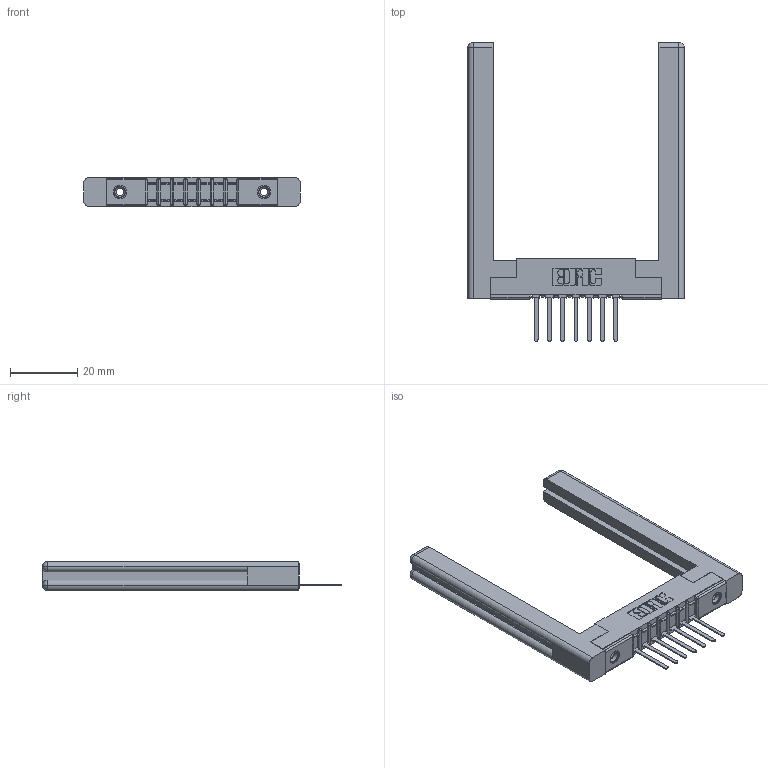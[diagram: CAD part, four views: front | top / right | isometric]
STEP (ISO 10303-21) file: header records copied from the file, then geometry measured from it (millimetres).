
FILE_DESCRIPTION (( 'STEP AP203' ), '1' );
FILE_NAME ('307-007-541-158.STEP', '2019-09-04T18:10:53', ( '' ), ( '' ), 'SwSTEP 2.0', 'SolidWorks 2016', '' );
FILE_SCHEMA (( 'CONFIG_CONTROL_DESIGN' ));
Length unit declared in the file: inch
Products named in the file (5): 345-250-001_345-250-001-102; 307 Part_.156 Dia Mounting Holes; 307-290-002_541; 307-007-541-158; 307-220-058
Assembly tree (12 placements, depth 2):
  307-007-541-158
    307 Part_.156 Dia Mounting Holes
    307-290-002_541  x7
    307-220-058  x2
    345-250-001_345-250-001-102  x2
Bounding box: 64.36 x 88.9 x 8.71 mm (x, y, z)
Volume: 11939.4 mm3; surface area: 12059.7 mm2
Topology: 12 solids, 12 shells, 786 faces, 2301 edges, 1498 vertices
Faces by surface type: plane 469, cylinder 277, sphere 16, torus 12, cone 12
Entity records: 13667 total; most frequent: CARTESIAN_POINT 2307, ORIENTED_EDGE 2236, DIRECTION 2218, EDGE_CURVE 1118, LINE 836, VECTOR 836, VERTEX_POINT 726, AXIS2_PLACEMENT_3D 691
